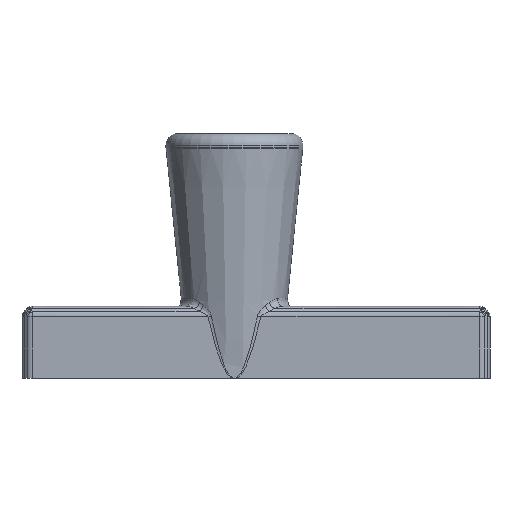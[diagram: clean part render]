
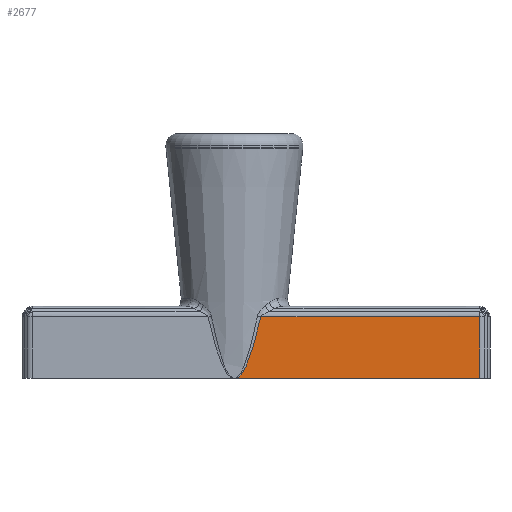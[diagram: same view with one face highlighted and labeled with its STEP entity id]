
A CAD part, front view. The second image highlights one B-rep face of the part: STEP entity #2677.
In plain terms, the highlighted planar face has unit normal (0, -1, 0).
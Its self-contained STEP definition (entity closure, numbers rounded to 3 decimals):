
#102=B_SPLINE_CURVE_WITH_KNOTS('',3,(#4917,#4918,#4919,#4920,#4921,#4922,
#4923,#4924),.UNSPECIFIED.,.F.,.F.,(4,1,1,1,1,4),(-3.399,-3.332,
-3.264,-3.13,-2.861,-2.458),
 .UNSPECIFIED.);
#146=PLANE('',#2995);
#374=FACE_OUTER_BOUND('',#557,.T.);
#557=EDGE_LOOP('',(#2354,#2355,#2356,#2357));
#675=LINE('',#4935,#850);
#710=LINE('',#5261,#885);
#725=LINE('',#5410,#900);
#850=VECTOR('',#3467,10.);
#885=VECTOR('',#3636,10.);
#900=VECTOR('',#3705,10.);
#1237=VERTEX_POINT('',#4818);
#1246=VERTEX_POINT('',#4873);
#1249=VERTEX_POINT('',#4915);
#1291=VERTEX_POINT('',#5257);
#1547=EDGE_CURVE('',#1249,#1246,#102,.T.);
#1550=EDGE_CURVE('',#1246,#1237,#675,.T.);
#1634=EDGE_CURVE('',#1237,#1291,#710,.T.);
#1659=EDGE_CURVE('',#1291,#1249,#725,.T.);
#2354=ORIENTED_EDGE('',*,*,#1547,.F.);
#2355=ORIENTED_EDGE('',*,*,#1659,.F.);
#2356=ORIENTED_EDGE('',*,*,#1634,.F.);
#2357=ORIENTED_EDGE('',*,*,#1550,.F.);
#2677=ADVANCED_FACE('',(#374),#146,.F.);
#2995=AXIS2_PLACEMENT_3D('',#5438,#3731,#3732);
#3467=DIRECTION('',(1.,0.,0.));
#3636=DIRECTION('',(0.,0.,-1.));
#3705=DIRECTION('',(-1.,0.,0.));
#3731=DIRECTION('center_axis',(0.,1.,0.));
#3732=DIRECTION('ref_axis',(0.,0.,
1.));
#4818=CARTESIAN_POINT('',(102.086,-56.25,14.936));
#4873=CARTESIAN_POINT('',(71.673,-56.25,14.936));
#4915=CARTESIAN_POINT('',(68.273,-56.25,6.35));
#4917=CARTESIAN_POINT('Ctrl Pts',(68.273,-56.25,6.35));
#4918=CARTESIAN_POINT('Ctrl Pts',(68.483,-56.25,6.428));
#4919=CARTESIAN_POINT('Ctrl Pts',(68.832,-56.25,6.725));
#4920=CARTESIAN_POINT('Ctrl Pts',(69.349,-56.25,7.463));
#4921=CARTESIAN_POINT('Ctrl Pts',(70.013,-56.25,8.883));
#4922=CARTESIAN_POINT('Ctrl Pts',(70.85,-56.25,11.461));
#4923=CARTESIAN_POINT('Ctrl Pts',(71.377,-56.25,13.62));
#4924=CARTESIAN_POINT('Ctrl Pts',(71.673,-56.25,14.936));
#4935=CARTESIAN_POINT('',(47.75,-56.25,14.936));
#5257=CARTESIAN_POINT('',(102.086,-56.25,6.35));
#5261=CARTESIAN_POINT('',(102.086,-56.25,5.837));
#5410=CARTESIAN_POINT('',(59.,-56.25,6.35));
#5438=CARTESIAN_POINT('Origin',(36.5,-56.25,5.666));
